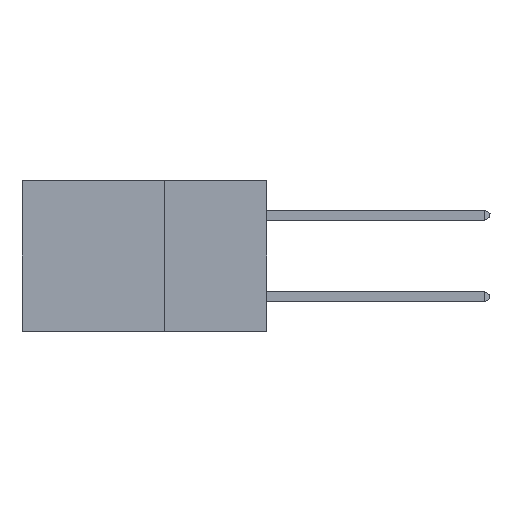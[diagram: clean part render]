
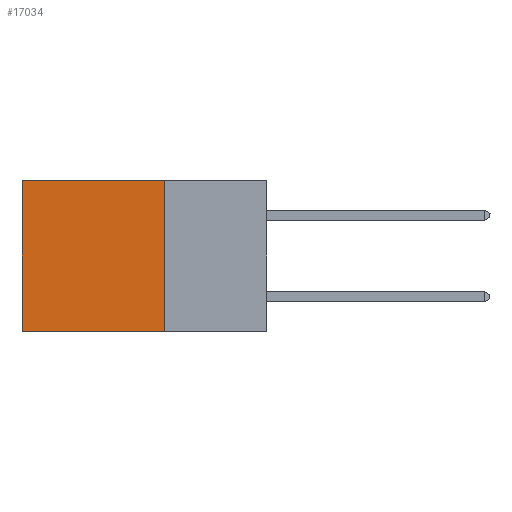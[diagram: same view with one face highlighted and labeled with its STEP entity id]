
A CAD part, left-side view. The second image highlights one B-rep face of the part: STEP entity #17034.
In plain terms, the highlighted planar face has unit normal (-1, 0, 0).
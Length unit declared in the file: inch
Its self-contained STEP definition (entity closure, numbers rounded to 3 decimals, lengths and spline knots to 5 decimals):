
#72 = ORIENTED_EDGE ( 'NONE', *, *, #1845, .F. ) ;
#431 = DIRECTION ( 'NONE',  ( 1., 0., 0. ) ) ;
#608 = VECTOR ( 'NONE', #7402, 39.37008 ) ;
#983 = CARTESIAN_POINT ( 'NONE',  ( 0.2875, 0.25, 0. ) ) ;
#1465 = LINE ( 'NONE', #14491, #608 ) ;
#1515 = DIRECTION ( 'NONE',  ( 0., 0., -1. ) ) ;
#1845 = EDGE_CURVE ( 'NONE', #9810, #9616, #14900, .T. ) ;
#1903 = VECTOR ( 'NONE', #15471, 39.37008 ) ;
#1951 = CARTESIAN_POINT ( 'NONE',  ( 0.2875, 0.25, 0. ) ) ;
#2920 = CARTESIAN_POINT ( 'NONE',  ( 0.2875, 0.6, 0. ) ) ;
#3001 = VERTEX_POINT ( 'NONE', #12849 ) ;
#5071 = CARTESIAN_POINT ( 'NONE',  ( 0.2875, 0.25, -0.37 ) ) ;
#5449 = VERTEX_POINT ( 'NONE', #11539 ) ;
#5512 = ORIENTED_EDGE ( 'NONE', *, *, #15637, .T. ) ;
#6676 = AXIS2_PLACEMENT_3D ( 'NONE', #1951, #431, #8961 ) ;
#7402 = DIRECTION ( 'NONE',  ( 0., 0., -1. ) ) ;
#7567 = LINE ( 'NONE', #2920, #10827 ) ;
#8300 = EDGE_LOOP ( 'NONE', ( #5512, #72, #14126, #12236 ) ) ;
#8346 = CARTESIAN_POINT ( 'NONE',  ( 0.2875, 0.6, -0.37 ) ) ;
#8961 = DIRECTION ( 'NONE',  ( 0., 0., -1. ) ) ;
#9616 = VERTEX_POINT ( 'NONE', #8346 ) ;
#9810 = VERTEX_POINT ( 'NONE', #5071 ) ;
#10262 = PLANE ( 'NONE',  #6676 ) ;
#10827 = VECTOR ( 'NONE', #1515, 39.37008 ) ;
#11539 = CARTESIAN_POINT ( 'NONE',  ( 0.2875, 0.25, 0. ) ) ;
#11605 = EDGE_CURVE ( 'NONE', #5449, #3001, #13082, .T. ) ;
#12236 = ORIENTED_EDGE ( 'NONE', *, *, #11605, .T. ) ;
#12640 = CARTESIAN_POINT ( 'NONE',  ( 0.2875, 0.25, -0.37 ) ) ;
#12687 = FACE_OUTER_BOUND ( 'NONE', #8300, .T. ) ;
#12849 = CARTESIAN_POINT ( 'NONE',  ( 0.2875, 0.6, 0. ) ) ;
#13082 = LINE ( 'NONE', #983, #15008 ) ;
#14126 = ORIENTED_EDGE ( 'NONE', *, *, #15796, .F. ) ;
#14491 = CARTESIAN_POINT ( 'NONE',  ( 0.2875, 0.25, 0. ) ) ;
#14900 = LINE ( 'NONE', #12640, #1903 ) ;
#15008 = VECTOR ( 'NONE', #16587, 39.37008 ) ;
#15471 = DIRECTION ( 'NONE',  ( 0., 1., 0. ) ) ;
#15637 = EDGE_CURVE ( 'NONE', #3001, #9616, #7567, .T. ) ;
#15796 = EDGE_CURVE ( 'NONE', #5449, #9810, #1465, .T. ) ;
#16587 = DIRECTION ( 'NONE',  ( 0., 1., 0. ) ) ;
#17034 = ADVANCED_FACE ( 'NONE', ( #12687 ), #10262, .F. ) ;
